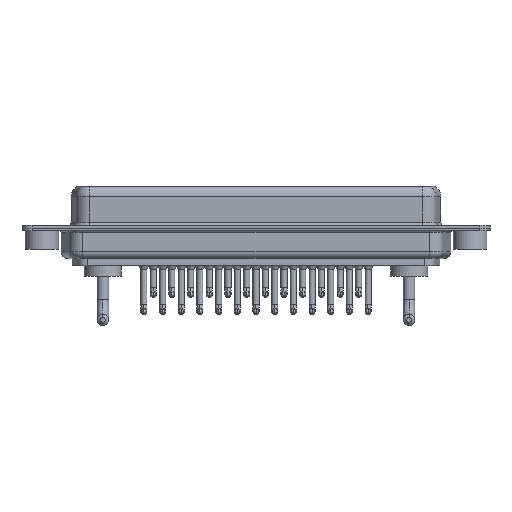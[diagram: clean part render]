
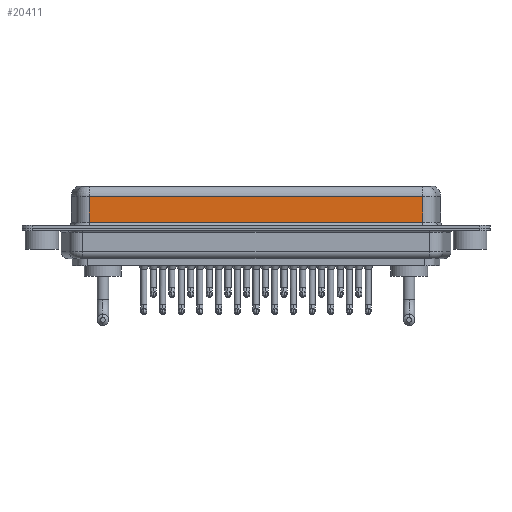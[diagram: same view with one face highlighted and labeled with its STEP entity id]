
A CAD part, front view. The second image highlights one B-rep face of the part: STEP entity #20411.
In plain terms, the highlighted planar face has unit normal (0, -1, 0).
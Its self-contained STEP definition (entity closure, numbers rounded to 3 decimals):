
#841 = LINE ( 'NONE', #14234, #18718 ) ;
#1477 = EDGE_CURVE ( 'NONE', #16635, #2310, #21837, .T. ) ;
#1665 = CARTESIAN_POINT ( 'NONE',  ( 56.462, -3.95, 6.4 ) ) ;
#2310 = VERTEX_POINT ( 'NONE', #24565 ) ;
#2820 = CARTESIAN_POINT ( 'NONE',  ( 7.038, -3.95, 0.9 ) ) ;
#3333 = ORIENTED_EDGE ( 'NONE', *, *, #19613, .F. ) ;
#4352 = DIRECTION ( 'NONE',  ( 0., 0., -1. ) ) ;
#4519 = VECTOR ( 'NONE', #9158, 1000. ) ;
#5294 = VERTEX_POINT ( 'NONE', #8279 ) ;
#6733 = AXIS2_PLACEMENT_3D ( 'NONE', #1665, #20853, #21096 ) ;
#7213 = EDGE_CURVE ( 'NONE', #22519, #5294, #8253, .T. ) ;
#7788 = FACE_OUTER_BOUND ( 'NONE', #8111, .T. ) ;
#8111 = EDGE_LOOP ( 'NONE', ( #3333, #17438, #23467, #19025 ) ) ;
#8253 = LINE ( 'NONE', #15914, #14811 ) ;
#8279 = CARTESIAN_POINT ( 'NONE',  ( 7.038, -3.95, 4.65 ) ) ;
#9158 = DIRECTION ( 'NONE',  ( 0., 0., -1. ) ) ;
#10910 = CARTESIAN_POINT ( 'NONE',  ( 7.038, -3.95, 6.4 ) ) ;
#13120 = EDGE_CURVE ( 'NONE', #5294, #16635, #22722, .T. ) ;
#13438 = PLANE ( 'NONE',  #6733 ) ;
#14029 = DIRECTION ( 'NONE',  ( -1., 0., 0. ) ) ;
#14234 = CARTESIAN_POINT ( 'NONE',  ( 56.462, -3.95, 6.4 ) ) ;
#14811 = VECTOR ( 'NONE', #14029, 1000. ) ;
#15914 = CARTESIAN_POINT ( 'NONE',  ( 56.462, -3.95, 4.65 ) ) ;
#15950 = CARTESIAN_POINT ( 'NONE',  ( 56.462, -3.95, 0.9 ) ) ;
#16635 = VERTEX_POINT ( 'NONE', #2820 ) ;
#17438 = ORIENTED_EDGE ( 'NONE', *, *, #7213, .T. ) ;
#17956 = DIRECTION ( 'NONE',  ( 1., 0., 0. ) ) ;
#18718 = VECTOR ( 'NONE', #4352, 1000. ) ;
#19025 = ORIENTED_EDGE ( 'NONE', *, *, #1477, .T. ) ;
#19433 = VECTOR ( 'NONE', #17956, 1000. ) ;
#19613 = EDGE_CURVE ( 'NONE', #22519, #2310, #841, .T. ) ;
#20411 = ADVANCED_FACE ( 'NONE', ( #7788 ), #13438, .F. ) ;
#20853 = DIRECTION ( 'NONE',  ( 0., 1., 0. ) ) ;
#21096 = DIRECTION ( 'NONE',  ( 0., 0., 1. ) ) ;
#21837 = LINE ( 'NONE', #15950, #19433 ) ;
#22519 = VERTEX_POINT ( 'NONE', #24398 ) ;
#22722 = LINE ( 'NONE', #10910, #4519 ) ;
#23467 = ORIENTED_EDGE ( 'NONE', *, *, #13120, .T. ) ;
#24398 = CARTESIAN_POINT ( 'NONE',  ( 56.462, -3.95, 4.65 ) ) ;
#24565 = CARTESIAN_POINT ( 'NONE',  ( 56.462, -3.95, 0.9 ) ) ;
